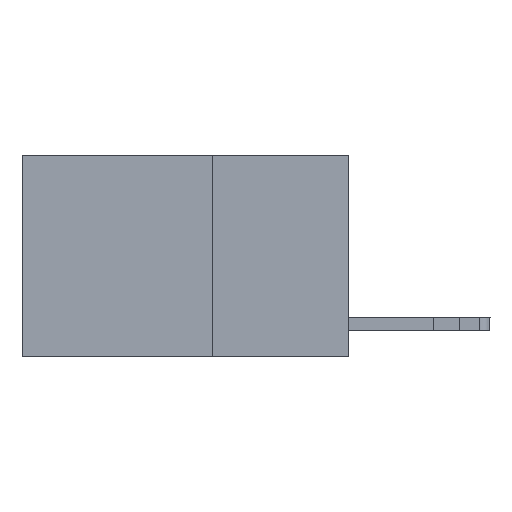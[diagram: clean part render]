
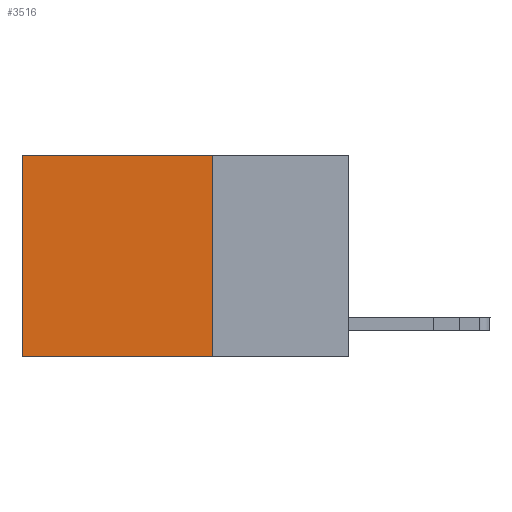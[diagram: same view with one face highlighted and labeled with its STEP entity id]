
A CAD part, left-side view. The second image highlights one B-rep face of the part: STEP entity #3516.
In plain terms, the highlighted planar face has unit normal (-1, 0, 0).
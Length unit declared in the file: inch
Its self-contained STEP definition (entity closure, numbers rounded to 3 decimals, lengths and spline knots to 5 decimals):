
#60 = CARTESIAN_POINT ( 'NONE',  ( 0.2625, 0.25, -0.37 ) ) ;
#454 = VECTOR ( 'NONE', #8609, 39.37008 ) ;
#720 = ORIENTED_EDGE ( 'NONE', *, *, #12371, .T. ) ;
#1162 = VERTEX_POINT ( 'NONE', #2668 ) ;
#1883 = VECTOR ( 'NONE', #10953, 39.37008 ) ;
#2040 = DIRECTION ( 'NONE',  ( 0., 0., -1. ) ) ;
#2668 = CARTESIAN_POINT ( 'NONE',  ( 0.2625, 0.25, 0. ) ) ;
#2829 = ORIENTED_EDGE ( 'NONE', *, *, #5664, .F. ) ;
#3329 = VECTOR ( 'NONE', #14797, 39.37008 ) ;
#3516 = ADVANCED_FACE ( 'NONE', ( #13656 ), #15058, .F. ) ;
#4222 = EDGE_CURVE ( 'NONE', #16556, #16028, #12302, .T. ) ;
#4597 = ORIENTED_EDGE ( 'NONE', *, *, #4908, .T. ) ;
#4908 = EDGE_CURVE ( 'NONE', #11222, #16028, #15792, .T. ) ;
#5624 = ORIENTED_EDGE ( 'NONE', *, *, #4222, .F. ) ;
#5664 = EDGE_CURVE ( 'NONE', #1162, #16556, #10131, .T. ) ;
#6774 = CARTESIAN_POINT ( 'NONE',  ( 0.2625, 0.6, -0.37 ) ) ;
#7372 = CARTESIAN_POINT ( 'NONE',  ( 0.2625, 0.25, 0. ) ) ;
#8032 = DIRECTION ( 'NONE',  ( 0., 0., -1. ) ) ;
#8466 = VECTOR ( 'NONE', #2040, 39.37008 ) ;
#8609 = DIRECTION ( 'NONE',  ( 0., 1., 0. ) ) ;
#9932 = CARTESIAN_POINT ( 'NONE',  ( 0.2625, 0.25, 0. ) ) ;
#10131 = LINE ( 'NONE', #7372, #8466 ) ;
#10953 = DIRECTION ( 'NONE',  ( 0., 1., 0. ) ) ;
#11096 = CARTESIAN_POINT ( 'NONE',  ( 0.2625, 0.25, -0.37 ) ) ;
#11222 = VERTEX_POINT ( 'NONE', #13470 ) ;
#11856 = AXIS2_PLACEMENT_3D ( 'NONE', #12223, #14879, #8032 ) ;
#12223 = CARTESIAN_POINT ( 'NONE',  ( 0.2625, 0.25, 0. ) ) ;
#12302 = LINE ( 'NONE', #60, #1883 ) ;
#12371 = EDGE_CURVE ( 'NONE', #1162, #11222, #14164, .T. ) ;
#13470 = CARTESIAN_POINT ( 'NONE',  ( 0.2625, 0.6, 0. ) ) ;
#13656 = FACE_OUTER_BOUND ( 'NONE', #14843, .T. ) ;
#14164 = LINE ( 'NONE', #9932, #454 ) ;
#14797 = DIRECTION ( 'NONE',  ( 0., 0., -1. ) ) ;
#14843 = EDGE_LOOP ( 'NONE', ( #4597, #5624, #2829, #720 ) ) ;
#14879 = DIRECTION ( 'NONE',  ( 1., 0., 0. ) ) ;
#15058 = PLANE ( 'NONE',  #11856 ) ;
#15792 = LINE ( 'NONE', #16393, #3329 ) ;
#16028 = VERTEX_POINT ( 'NONE', #6774 ) ;
#16393 = CARTESIAN_POINT ( 'NONE',  ( 0.2625, 0.6, 0. ) ) ;
#16556 = VERTEX_POINT ( 'NONE', #11096 ) ;
